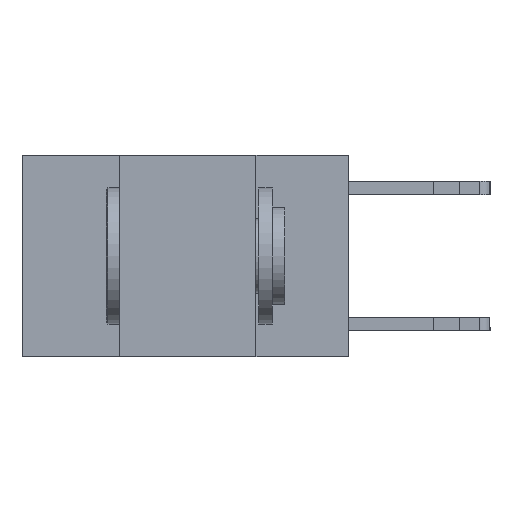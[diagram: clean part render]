
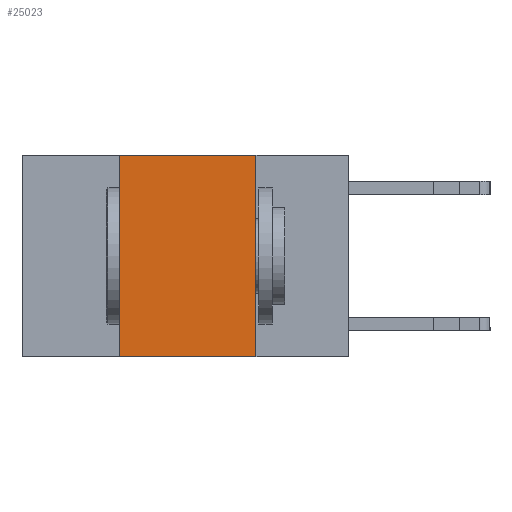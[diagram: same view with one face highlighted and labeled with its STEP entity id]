
A CAD part, left-side view. The second image highlights one B-rep face of the part: STEP entity #25023.
In plain terms, the highlighted planar face has unit normal (-1, 0, 0).
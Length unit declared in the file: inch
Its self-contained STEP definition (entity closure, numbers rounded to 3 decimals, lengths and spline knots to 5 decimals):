
#272 = LINE ( 'NONE', #2029, #28474 ) ;
#2029 = CARTESIAN_POINT ( 'NONE',  ( 0., 0.42, 0. ) ) ;
#2755 = CARTESIAN_POINT ( 'NONE',  ( 0., 0.6, 0. ) ) ;
#3037 = DIRECTION ( 'NONE',  ( 0., -1., 0. ) ) ;
#4449 = AXIS2_PLACEMENT_3D ( 'NONE', #16869, #8321, #17154 ) ;
#6146 = VERTEX_POINT ( 'NONE', #21741 ) ;
#6991 = CARTESIAN_POINT ( 'NONE',  ( 0., 0.6, -0.37 ) ) ;
#7846 = ORIENTED_EDGE ( 'NONE', *, *, #9325, .F. ) ;
#7849 = ORIENTED_EDGE ( 'NONE', *, *, #22790, .F. ) ;
#8240 = VERTEX_POINT ( 'NONE', #26935 ) ;
#8321 = DIRECTION ( 'NONE',  ( 1., 0., 0. ) ) ;
#9325 = EDGE_CURVE ( 'NONE', #26462, #20677, #20458, .T. ) ;
#9574 = CARTESIAN_POINT ( 'NONE',  ( 0., 0.17, 0. ) ) ;
#10303 = ORIENTED_EDGE ( 'NONE', *, *, #20882, .T. ) ;
#10627 = PLANE ( 'NONE',  #4449 ) ;
#11309 = VECTOR ( 'NONE', #19757, 39.37008 ) ;
#13914 = LINE ( 'NONE', #2755, #18420 ) ;
#16239 = EDGE_LOOP ( 'NONE', ( #7846, #20042, #7849, #10303 ) ) ;
#16869 = CARTESIAN_POINT ( 'NONE',  ( 0., 0.6, 0. ) ) ;
#17154 = DIRECTION ( 'NONE',  ( 0., 0., -1. ) ) ;
#17396 = DIRECTION ( 'NONE',  ( 0., 0., 1. ) ) ;
#18420 = VECTOR ( 'NONE', #3037, 39.37008 ) ;
#19757 = DIRECTION ( 'NONE',  ( 0., -1., 0. ) ) ;
#19906 = LINE ( 'NONE', #6991, #11309 ) ;
#20042 = ORIENTED_EDGE ( 'NONE', *, *, #26967, .F. ) ;
#20458 = LINE ( 'NONE', #9574, #23237 ) ;
#20677 = VERTEX_POINT ( 'NONE', #25017 ) ;
#20882 = EDGE_CURVE ( 'NONE', #6146, #20677, #19906, .T. ) ;
#21741 = CARTESIAN_POINT ( 'NONE',  ( 0., 0.42, -0.37 ) ) ;
#22790 = EDGE_CURVE ( 'NONE', #6146, #8240, #272, .T. ) ;
#23237 = VECTOR ( 'NONE', #24829, 39.37008 ) ;
#23409 = FACE_OUTER_BOUND ( 'NONE', #16239, .T. ) ;
#24829 = DIRECTION ( 'NONE',  ( 0., 0., -1. ) ) ;
#25017 = CARTESIAN_POINT ( 'NONE',  ( 0., 0.17, -0.37 ) ) ;
#25023 = ADVANCED_FACE ( 'NONE', ( #23409 ), #10627, .F. ) ;
#26028 = CARTESIAN_POINT ( 'NONE',  ( 0., 0.17, 0. ) ) ;
#26462 = VERTEX_POINT ( 'NONE', #26028 ) ;
#26935 = CARTESIAN_POINT ( 'NONE',  ( 0., 0.42, 0. ) ) ;
#26967 = EDGE_CURVE ( 'NONE', #8240, #26462, #13914, .T. ) ;
#28474 = VECTOR ( 'NONE', #17396, 39.37008 ) ;
